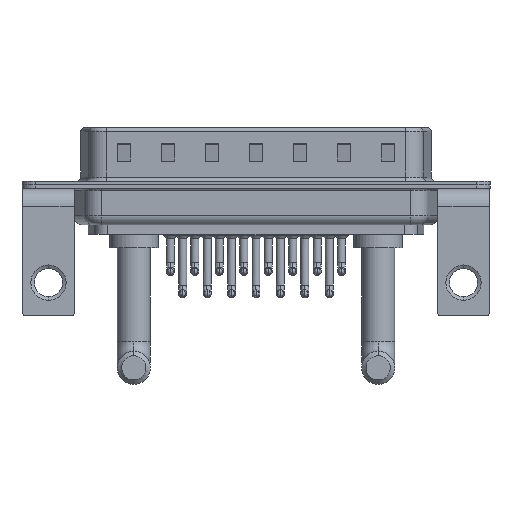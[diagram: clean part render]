
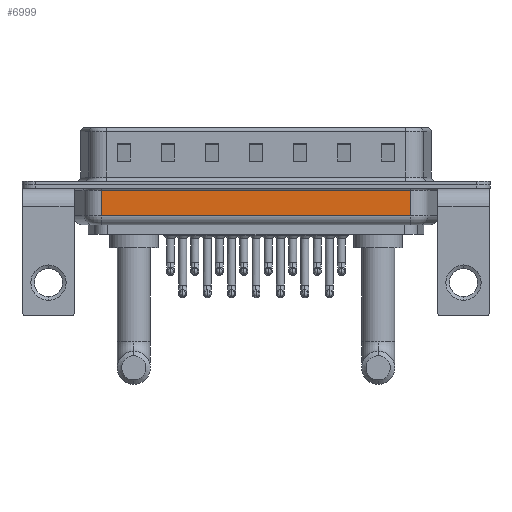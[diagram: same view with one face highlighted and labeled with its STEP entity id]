
A CAD part, front view. The second image highlights one B-rep face of the part: STEP entity #6999.
In plain terms, the highlighted planar face has unit normal (0, -1, 0).
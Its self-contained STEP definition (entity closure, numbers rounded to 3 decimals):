
#1558 = CARTESIAN_POINT ( 'NONE',  ( 6.006, -5.35, -0.65 ) ) ;
#2119 = DIRECTION ( 'NONE',  ( 1., 0., 0. ) ) ;
#2426 = AXIS2_PLACEMENT_3D ( 'NONE', #25205, #15205, #21545 ) ;
#3218 = CARTESIAN_POINT ( 'NONE',  ( 6.006, -5.35, -4.5 ) ) ;
#4075 = CARTESIAN_POINT ( 'NONE',  ( 6.006, -5.35, -3.5 ) ) ;
#4210 = VERTEX_POINT ( 'NONE', #22729 ) ;
#5030 = DIRECTION ( 'NONE',  ( 0., 0., 1. ) ) ;
#5458 = FACE_OUTER_BOUND ( 'NONE', #10109, .T. ) ;
#6440 = ORIENTED_EDGE ( 'NONE', *, *, #10001, .T. ) ;
#6959 = VERTEX_POINT ( 'NONE', #1558 ) ;
#6999 = ADVANCED_FACE ( 'NONE', ( #5458 ), #19226, .F. ) ;
#7107 = LINE ( 'NONE', #3218, #22911 ) ;
#7253 = VECTOR ( 'NONE', #11541, 1000. ) ;
#8460 = VERTEX_POINT ( 'NONE', #14414 ) ;
#10001 = EDGE_CURVE ( 'NONE', #4210, #6959, #11806, .T. ) ;
#10109 = EDGE_LOOP ( 'NONE', ( #13099, #25047, #23478, #6440 ) ) ;
#10130 = LINE ( 'NONE', #14161, #21391 ) ;
#10878 = EDGE_CURVE ( 'NONE', #8460, #4210, #10130, .T. ) ;
#11541 = DIRECTION ( 'NONE',  ( -1., 0., 0. ) ) ;
#11668 = CARTESIAN_POINT ( 'NONE',  ( 6.006, -5.35, -0.65 ) ) ;
#11806 = LINE ( 'NONE', #11668, #7253 ) ;
#11906 = CARTESIAN_POINT ( 'NONE',  ( 6.006, -5.35, -3.5 ) ) ;
#12265 = LINE ( 'NONE', #4075, #14247 ) ;
#13099 = ORIENTED_EDGE ( 'NONE', *, *, #23164, .F. ) ;
#14161 = CARTESIAN_POINT ( 'NONE',  ( 41.044, -5.35, -4.5 ) ) ;
#14247 = VECTOR ( 'NONE', #2119, 1000. ) ;
#14414 = CARTESIAN_POINT ( 'NONE',  ( 41.044, -5.35, -3.5 ) ) ;
#15205 = DIRECTION ( 'NONE',  ( 0., 1., 0. ) ) ;
#18077 = VERTEX_POINT ( 'NONE', #11906 ) ;
#19226 = PLANE ( 'NONE',  #2426 ) ;
#21391 = VECTOR ( 'NONE', #21554, 1000. ) ;
#21545 = DIRECTION ( 'NONE',  ( 0., 0., 1. ) ) ;
#21554 = DIRECTION ( 'NONE',  ( 0., 0., 1. ) ) ;
#22729 = CARTESIAN_POINT ( 'NONE',  ( 41.044, -5.35, -0.65 ) ) ;
#22911 = VECTOR ( 'NONE', #5030, 1000. ) ;
#23164 = EDGE_CURVE ( 'NONE', #18077, #6959, #7107, .T. ) ;
#23478 = ORIENTED_EDGE ( 'NONE', *, *, #10878, .T. ) ;
#23952 = EDGE_CURVE ( 'NONE', #18077, #8460, #12265, .T. ) ;
#25047 = ORIENTED_EDGE ( 'NONE', *, *, #23952, .T. ) ;
#25205 = CARTESIAN_POINT ( 'NONE',  ( 6.006, -5.35, -4.5 ) ) ;
